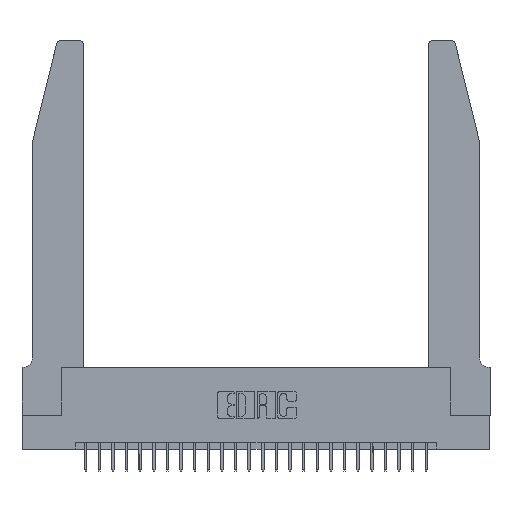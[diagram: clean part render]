
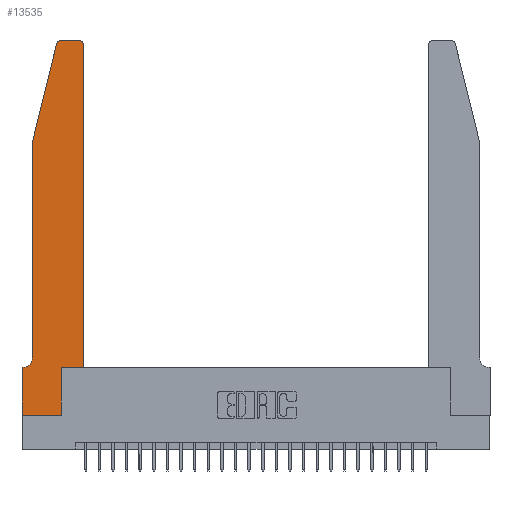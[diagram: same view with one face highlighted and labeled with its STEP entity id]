
A CAD part, top view. The second image highlights one B-rep face of the part: STEP entity #13535.
In plain terms, the highlighted planar face has unit normal (0, 0, 1).
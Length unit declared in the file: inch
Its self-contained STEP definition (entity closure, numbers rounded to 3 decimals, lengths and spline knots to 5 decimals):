
#224 = CARTESIAN_POINT ( 'NONE',  ( 0., 0.35, 0.37 ) ) ;
#450 = VERTEX_POINT ( 'NONE', #3966 ) ;
#764 = DIRECTION ( 'NONE',  ( 1., 0., 0. ) ) ;
#779 = VERTEX_POINT ( 'NONE', #13037 ) ;
#1478 = CARTESIAN_POINT ( 'NONE',  ( 0.0055, 0.42, 0.37 ) ) ;
#1974 = VERTEX_POINT ( 'NONE', #18621 ) ;
#2019 = ORIENTED_EDGE ( 'NONE', *, *, #11546, .T. ) ;
#2353 = DIRECTION ( 'NONE',  ( 0., -1., 0. ) ) ;
#2537 = CARTESIAN_POINT ( 'NONE',  ( 0.0755, 2., 0.37 ) ) ;
#2568 = PLANE ( 'NONE',  #7763 ) ;
#2723 = DIRECTION ( 'NONE',  ( 1., 0., 0. ) ) ;
#2833 = ORIENTED_EDGE ( 'NONE', *, *, #5369, .T. ) ;
#3603 = DIRECTION ( 'NONE',  ( 1., 0., 0. ) ) ;
#3692 = AXIS2_PLACEMENT_3D ( 'NONE', #7237, #11398, #764 ) ;
#3763 = EDGE_CURVE ( 'NONE', #20974, #12237, #11195, .T. ) ;
#3966 = CARTESIAN_POINT ( 'NONE',  ( 0.4505, 0.35, 0.37 ) ) ;
#4545 = ORIENTED_EDGE ( 'NONE', *, *, #14241, .T. ) ;
#4689 = DIRECTION ( 'NONE',  ( 1., 0., 0. ) ) ;
#4997 = EDGE_CURVE ( 'NONE', #10170, #20974, #15584, .T. ) ;
#5146 = CARTESIAN_POINT ( 'NONE',  ( 0.2865, 0.35, 0.37 ) ) ;
#5369 = EDGE_CURVE ( 'NONE', #8040, #450, #25848, .T. ) ;
#5472 = DIRECTION ( 'NONE',  ( 0., 0., -1. ) ) ;
#5633 = VERTEX_POINT ( 'NONE', #17494 ) ;
#7237 = CARTESIAN_POINT ( 'NONE',  ( 0.284, 2.72, 0.37 ) ) ;
#7580 = DIRECTION ( 'NONE',  ( -1., 0., 0. ) ) ;
#7763 = AXIS2_PLACEMENT_3D ( 'NONE', #224, #23738, #4689 ) ;
#7806 = AXIS2_PLACEMENT_3D ( 'NONE', #1478, #5472, #7580 ) ;
#8040 = VERTEX_POINT ( 'NONE', #16398 ) ;
#8459 = LINE ( 'NONE', #23966, #12119 ) ;
#8781 = CARTESIAN_POINT ( 'NONE',  ( 0.0055, 0.35, 0.37 ) ) ;
#8789 = LINE ( 'NONE', #18923, #19392 ) ;
#8812 = VERTEX_POINT ( 'NONE', #26756 ) ;
#9110 = ORIENTED_EDGE ( 'NONE', *, *, #21999, .T. ) ;
#9852 = EDGE_LOOP ( 'NONE', ( #26914, #16032, #2019, #24779, #13712, #18540, #15418, #4545, #9110, #2833, #19905, #12933 ) ) ;
#10170 = VERTEX_POINT ( 'NONE', #26617 ) ;
#10232 = DIRECTION ( 'NONE',  ( 0., 0., 1. ) ) ;
#10609 = CIRCLE ( 'NONE', #17391, 0.03 ) ;
#10672 = EDGE_CURVE ( 'NONE', #450, #779, #19929, .T. ) ;
#11195 = CIRCLE ( 'NONE', #7806, 0.07 ) ;
#11197 = CARTESIAN_POINT ( 'NONE',  ( 0., 0., 0.37 ) ) ;
#11398 = DIRECTION ( 'NONE',  ( 0., 0., 1. ) ) ;
#11461 = CARTESIAN_POINT ( 'NONE',  ( 0.4505, 0.35, 0.37 ) ) ;
#11546 = EDGE_CURVE ( 'NONE', #17502, #10170, #8789, .T. ) ;
#12119 = VECTOR ( 'NONE', #26464, 39.37008 ) ;
#12237 = VERTEX_POINT ( 'NONE', #8781 ) ;
#12933 = ORIENTED_EDGE ( 'NONE', *, *, #15273, .T. ) ;
#12947 = VECTOR ( 'NONE', #2353, 39.37008 ) ;
#13037 = CARTESIAN_POINT ( 'NONE',  ( 0.4505, 2.72, 0.37 ) ) ;
#13535 = ADVANCED_FACE ( 'NONE', ( #19959 ), #2568, .T. ) ;
#13712 = ORIENTED_EDGE ( 'NONE', *, *, #3763, .T. ) ;
#13732 = CARTESIAN_POINT ( 'NONE',  ( 0.4505, 0.35, 0.37 ) ) ;
#14241 = EDGE_CURVE ( 'NONE', #5633, #8812, #25584, .T. ) ;
#14700 = VECTOR ( 'NONE', #21949, 39.37008 ) ;
#15030 = DIRECTION ( 'NONE',  ( -1., 0., 0. ) ) ;
#15273 = EDGE_CURVE ( 'NONE', #779, #25448, #10609, .T. ) ;
#15418 = ORIENTED_EDGE ( 'NONE', *, *, #20443, .T. ) ;
#15562 = CARTESIAN_POINT ( 'NONE',  ( 0., 0., 0.37 ) ) ;
#15584 = LINE ( 'NONE', #2537, #12947 ) ;
#15601 = CARTESIAN_POINT ( 'NONE',  ( 0., 0.35, 0.37 ) ) ;
#15760 = DIRECTION ( 'NONE',  ( 0., 1., 0. ) ) ;
#15768 = DIRECTION ( 'NONE',  ( 0., 1., 0. ) ) ;
#16032 = ORIENTED_EDGE ( 'NONE', *, *, #20438, .T. ) ;
#16398 = CARTESIAN_POINT ( 'NONE',  ( 0.2865, 0.35, 0.37 ) ) ;
#16720 = CARTESIAN_POINT ( 'NONE',  ( 0.4205, 2.72, 0.37 ) ) ;
#17391 = AXIS2_PLACEMENT_3D ( 'NONE', #16720, #10232, #27173 ) ;
#17392 = EDGE_CURVE ( 'NONE', #12237, #19839, #18769, .T. ) ;
#17494 = CARTESIAN_POINT ( 'NONE',  ( 0., 0., 0.37 ) ) ;
#17502 = VERTEX_POINT ( 'NONE', #17732 ) ;
#17732 = CARTESIAN_POINT ( 'NONE',  ( 0.25487, 2.72718, 0.37 ) ) ;
#18044 = CIRCLE ( 'NONE', #3692, 0.03 ) ;
#18540 = ORIENTED_EDGE ( 'NONE', *, *, #17392, .T. ) ;
#18621 = CARTESIAN_POINT ( 'NONE',  ( 0.284, 2.75, 0.37 ) ) ;
#18769 = LINE ( 'NONE', #21589, #23740 ) ;
#18923 = CARTESIAN_POINT ( 'NONE',  ( 0.0755, 2., 0.37 ) ) ;
#19062 = CARTESIAN_POINT ( 'NONE',  ( 0.0755, 0.42, 0.37 ) ) ;
#19392 = VECTOR ( 'NONE', #20868, 39.37008 ) ;
#19839 = VERTEX_POINT ( 'NONE', #15601 ) ;
#19905 = ORIENTED_EDGE ( 'NONE', *, *, #10672, .T. ) ;
#19929 = LINE ( 'NONE', #13732, #22588 ) ;
#19959 = FACE_OUTER_BOUND ( 'NONE', #9852, .T. ) ;
#20331 = LINE ( 'NONE', #15562, #14700 ) ;
#20438 = EDGE_CURVE ( 'NONE', #1974, #17502, #18044, .T. ) ;
#20443 = EDGE_CURVE ( 'NONE', #19839, #5633, #20331, .T. ) ;
#20868 = DIRECTION ( 'NONE',  ( -0.239, -0.971, 0. ) ) ;
#20974 = VERTEX_POINT ( 'NONE', #19062 ) ;
#21589 = CARTESIAN_POINT ( 'NONE',  ( 0.0755, 0.35, 0.37 ) ) ;
#21949 = DIRECTION ( 'NONE',  ( 0., -1., 0. ) ) ;
#21999 = EDGE_CURVE ( 'NONE', #8812, #8040, #27167, .T. ) ;
#22506 = CARTESIAN_POINT ( 'NONE',  ( 0.4205, 2.75, 0.37 ) ) ;
#22588 = VECTOR ( 'NONE', #15760, 39.37008 ) ;
#23407 = EDGE_CURVE ( 'NONE', #25448, #1974, #8459, .T. ) ;
#23738 = DIRECTION ( 'NONE',  ( 0., 0., 1. ) ) ;
#23740 = VECTOR ( 'NONE', #15030, 39.37008 ) ;
#23966 = CARTESIAN_POINT ( 'NONE',  ( 0.2605, 2.75, 0.37 ) ) ;
#24208 = VECTOR ( 'NONE', #15768, 39.37008 ) ;
#24529 = VECTOR ( 'NONE', #3603, 39.37008 ) ;
#24779 = ORIENTED_EDGE ( 'NONE', *, *, #4997, .T. ) ;
#25448 = VERTEX_POINT ( 'NONE', #22506 ) ;
#25584 = LINE ( 'NONE', #11197, #26592 ) ;
#25848 = LINE ( 'NONE', #11461, #24529 ) ;
#26464 = DIRECTION ( 'NONE',  ( -1., 0., 0. ) ) ;
#26592 = VECTOR ( 'NONE', #2723, 39.37008 ) ;
#26617 = CARTESIAN_POINT ( 'NONE',  ( 0.0755, 2., 0.37 ) ) ;
#26756 = CARTESIAN_POINT ( 'NONE',  ( 0.2865, 0., 0.37 ) ) ;
#26914 = ORIENTED_EDGE ( 'NONE', *, *, #23407, .T. ) ;
#27167 = LINE ( 'NONE', #5146, #24208 ) ;
#27173 = DIRECTION ( 'NONE',  ( 1., 0., 0. ) ) ;
